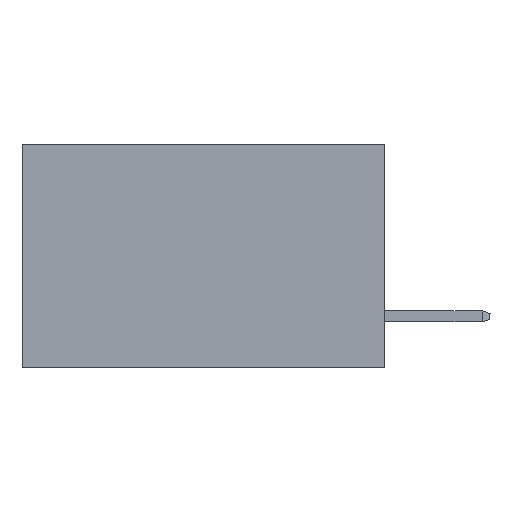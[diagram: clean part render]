
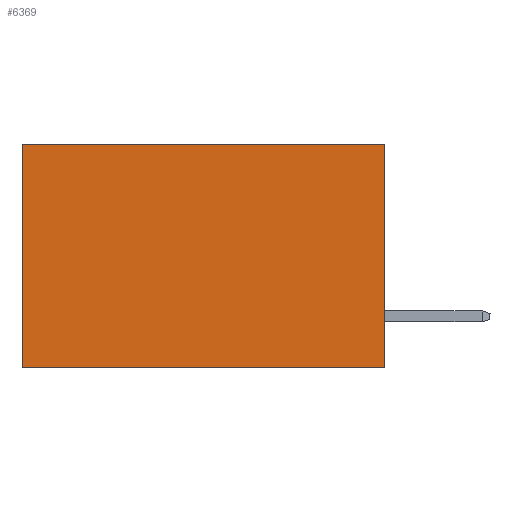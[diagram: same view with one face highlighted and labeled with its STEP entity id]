
A CAD part, left-side view. The second image highlights one B-rep face of the part: STEP entity #6369.
In plain terms, the highlighted planar face has unit normal (-1, 0, 0).
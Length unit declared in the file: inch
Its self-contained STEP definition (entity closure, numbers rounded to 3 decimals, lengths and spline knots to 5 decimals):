
#472 = CARTESIAN_POINT ( 'NONE',  ( 0.2615, 0., -0.37 ) ) ;
#1114 = EDGE_CURVE ( 'NONE', #18920, #6814, #14786, .T. ) ;
#1719 = CARTESIAN_POINT ( 'NONE',  ( 0.2615, 0.6, 0. ) ) ;
#2734 = ORIENTED_EDGE ( 'NONE', *, *, #11185, .T. ) ;
#3107 = CARTESIAN_POINT ( 'NONE',  ( 0.2615, 0.6, -0.37 ) ) ;
#3194 = CARTESIAN_POINT ( 'NONE',  ( 0.2615, 0., 0. ) ) ;
#3638 = CARTESIAN_POINT ( 'NONE',  ( 0.2615, 0.6, -0.37 ) ) ;
#4367 = VECTOR ( 'NONE', #19831, 39.37008 ) ;
#5310 = DIRECTION ( 'NONE',  ( 0., 1., 0. ) ) ;
#5547 = DIRECTION ( 'NONE',  ( 1., 0., 0. ) ) ;
#6369 = ADVANCED_FACE ( 'NONE', ( #12228 ), #16713, .F. ) ;
#6659 = LINE ( 'NONE', #3194, #17556 ) ;
#6814 = VERTEX_POINT ( 'NONE', #12309 ) ;
#6982 = EDGE_CURVE ( 'NONE', #18920, #14090, #6659, .T. ) ;
#7523 = ORIENTED_EDGE ( 'NONE', *, *, #12414, .F. ) ;
#8112 = VERTEX_POINT ( 'NONE', #3107 ) ;
#8233 = CARTESIAN_POINT ( 'NONE',  ( 0.2615, 0., -0.37 ) ) ;
#8896 = CARTESIAN_POINT ( 'NONE',  ( 0.2615, 0., -0.37 ) ) ;
#11185 = EDGE_CURVE ( 'NONE', #14090, #8112, #19616, .T. ) ;
#12224 = VECTOR ( 'NONE', #5310, 39.37008 ) ;
#12228 = FACE_OUTER_BOUND ( 'NONE', #17308, .T. ) ;
#12309 = CARTESIAN_POINT ( 'NONE',  ( 0.2615, 0., -0.37 ) ) ;
#12414 = EDGE_CURVE ( 'NONE', #6814, #8112, #14791, .T. ) ;
#12884 = CARTESIAN_POINT ( 'NONE',  ( 0.2615, 0., 0. ) ) ;
#13014 = DIRECTION ( 'NONE',  ( 0., 1., 0. ) ) ;
#13266 = AXIS2_PLACEMENT_3D ( 'NONE', #8896, #5547, #15234 ) ;
#14090 = VERTEX_POINT ( 'NONE', #1719 ) ;
#14690 = DIRECTION ( 'NONE',  ( 0., 0., -1. ) ) ;
#14786 = LINE ( 'NONE', #8233, #4367 ) ;
#14791 = LINE ( 'NONE', #472, #12224 ) ;
#14826 = ORIENTED_EDGE ( 'NONE', *, *, #6982, .T. ) ;
#15221 = ORIENTED_EDGE ( 'NONE', *, *, #1114, .F. ) ;
#15234 = DIRECTION ( 'NONE',  ( 0., 0., -1. ) ) ;
#15674 = VECTOR ( 'NONE', #14690, 39.37008 ) ;
#16713 = PLANE ( 'NONE',  #13266 ) ;
#17308 = EDGE_LOOP ( 'NONE', ( #2734, #7523, #15221, #14826 ) ) ;
#17556 = VECTOR ( 'NONE', #13014, 39.37008 ) ;
#18920 = VERTEX_POINT ( 'NONE', #12884 ) ;
#19616 = LINE ( 'NONE', #3638, #15674 ) ;
#19831 = DIRECTION ( 'NONE',  ( 0., 0., -1. ) ) ;
